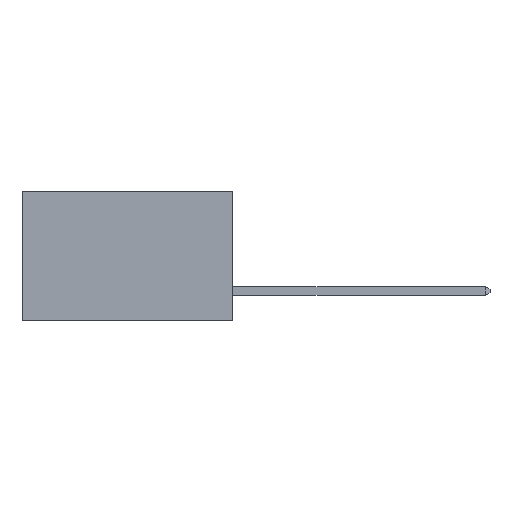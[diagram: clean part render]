
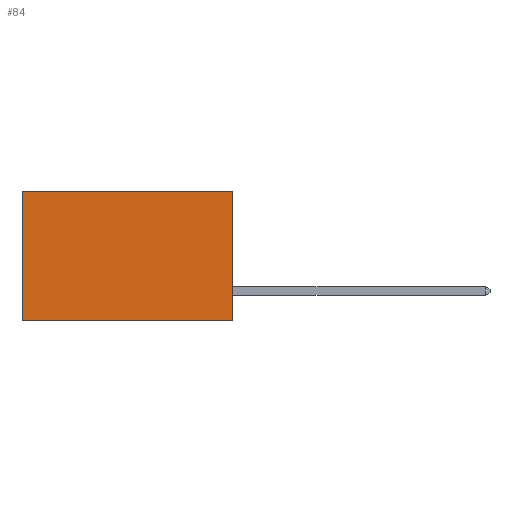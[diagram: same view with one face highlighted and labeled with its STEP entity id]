
A CAD part, left-side view. The second image highlights one B-rep face of the part: STEP entity #84.
In plain terms, the highlighted planar face has unit normal (-1, 0, 0).
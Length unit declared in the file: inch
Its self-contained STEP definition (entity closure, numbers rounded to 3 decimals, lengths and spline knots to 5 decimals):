
#13 = ORIENTED_EDGE ( 'NONE', *, *, #4495, .F. ) ;
#84 = ADVANCED_FACE ( 'NONE', ( #3507 ), #5653, .F. ) ;
#643 = DIRECTION ( 'NONE',  ( 0., 0., -1. ) ) ;
#996 = CARTESIAN_POINT ( 'NONE',  ( 0.2875, 0., -0.37 ) ) ;
#1560 = EDGE_CURVE ( 'NONE', #5888, #10528, #8901, .T. ) ;
#1733 = EDGE_CURVE ( 'NONE', #6769, #9429, #9513, .T. ) ;
#2034 = DIRECTION ( 'NONE',  ( 0., 0., -1. ) ) ;
#2795 = CARTESIAN_POINT ( 'NONE',  ( 0.2875, 0.6, 0. ) ) ;
#3507 = FACE_OUTER_BOUND ( 'NONE', #9714, .T. ) ;
#3698 = VECTOR ( 'NONE', #5103, 39.37008 ) ;
#4039 = ORIENTED_EDGE ( 'NONE', *, *, #1560, .T. ) ;
#4495 = EDGE_CURVE ( 'NONE', #9429, #10528, #9332, .T. ) ;
#4721 = CARTESIAN_POINT ( 'NONE',  ( 0.2875, 0., 0. ) ) ;
#4749 = VECTOR ( 'NONE', #11011, 39.37008 ) ;
#5103 = DIRECTION ( 'NONE',  ( 0., 1., 0. ) ) ;
#5586 = DIRECTION ( 'NONE',  ( 1., 0., 0. ) ) ;
#5653 = PLANE ( 'NONE',  #6760 ) ;
#5860 = LINE ( 'NONE', #6699, #3698 ) ;
#5888 = VERTEX_POINT ( 'NONE', #10423 ) ;
#5929 = DIRECTION ( 'NONE',  ( 0., 0., -1. ) ) ;
#5948 = CARTESIAN_POINT ( 'NONE',  ( 0.2875, 0., 0. ) ) ;
#5983 = EDGE_CURVE ( 'NONE', #6769, #5888, #5860, .T. ) ;
#6699 = CARTESIAN_POINT ( 'NONE',  ( 0.2875, 0., 0. ) ) ;
#6760 = AXIS2_PLACEMENT_3D ( 'NONE', #10710, #5586, #2034 ) ;
#6769 = VERTEX_POINT ( 'NONE', #5948 ) ;
#8426 = ORIENTED_EDGE ( 'NONE', *, *, #1733, .F. ) ;
#8901 = LINE ( 'NONE', #2795, #11223 ) ;
#9332 = LINE ( 'NONE', #10982, #4749 ) ;
#9429 = VERTEX_POINT ( 'NONE', #996 ) ;
#9513 = LINE ( 'NONE', #4721, #11326 ) ;
#9714 = EDGE_LOOP ( 'NONE', ( #4039, #13, #8426, #10574 ) ) ;
#10249 = CARTESIAN_POINT ( 'NONE',  ( 0.2875, 0.6, -0.37 ) ) ;
#10423 = CARTESIAN_POINT ( 'NONE',  ( 0.2875, 0.6, 0. ) ) ;
#10528 = VERTEX_POINT ( 'NONE', #10249 ) ;
#10574 = ORIENTED_EDGE ( 'NONE', *, *, #5983, .T. ) ;
#10710 = CARTESIAN_POINT ( 'NONE',  ( 0.2875, 0., 0. ) ) ;
#10982 = CARTESIAN_POINT ( 'NONE',  ( 0.2875, 0., -0.37 ) ) ;
#11011 = DIRECTION ( 'NONE',  ( 0., 1., 0. ) ) ;
#11223 = VECTOR ( 'NONE', #5929, 39.37008 ) ;
#11326 = VECTOR ( 'NONE', #643, 39.37008 ) ;
